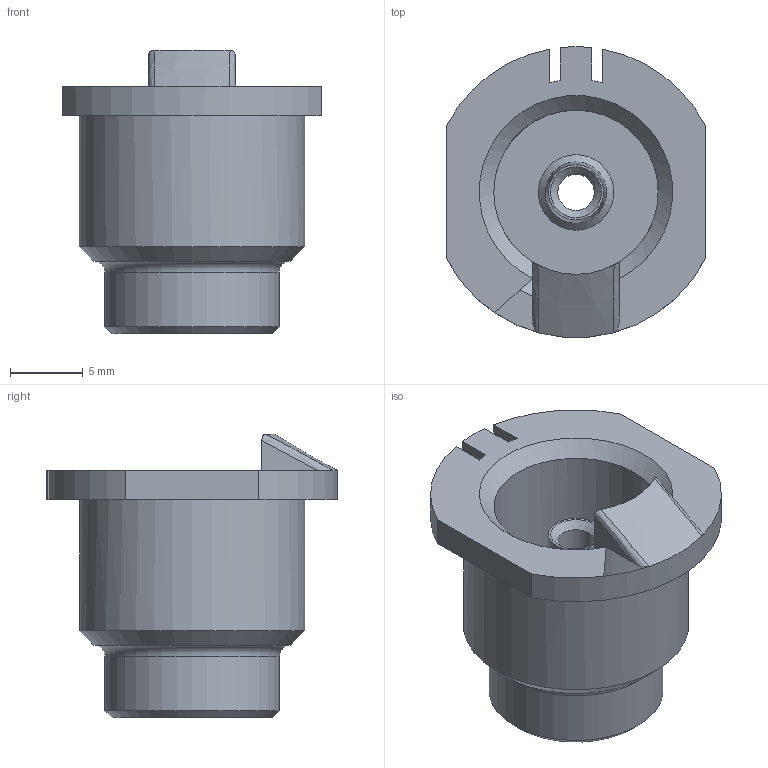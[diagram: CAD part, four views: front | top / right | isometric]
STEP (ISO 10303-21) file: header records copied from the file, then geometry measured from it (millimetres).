
FILE_DESCRIPTION(/* description */ (''),/* implementation_level */ '2;1');
FILE_NAME(/* name */ 'Fuse Base.step',/* time_stamp */ '2020-10-22T17:43:10-04:00',/* author */ (''),/* organization */ (''),/* preprocessor_version */ 'ST-DEVELOPER v18.1',/* originating_system */ 'Autodesk Translation Framework v9.3.0.1241',/* authorisation */ '');
FILE_SCHEMA (('AUTOMOTIVE_DESIGN { 1 0 10303 214 3 1 1 }'));
Length unit declared in the file: millimetre
Products named in the file (1): Fuse Base
Bounding box: 17.79 x 19.96 x 19.5 mm (x, y, z)
Volume: 1930.8 mm3; surface area: 1948.9 mm2
Topology: 1 solids, 1 shells, 44 faces, 111 edges, 72 vertices
Faces by surface type: plane 19, cylinder 12, cone 10, bspline 2, torus 1
Full cylindrical faces by diameter (mm): 2.5 x1, 3 x1, 4.191 x1, 6 x1, 11.3 x1, 12 x1, 15.5 x1
Entity records: 1494 total; most frequent: CARTESIAN_POINT 378, DIRECTION 235, ORIENTED_EDGE 222, EDGE_CURVE 111, AXIS2_PLACEMENT_3D 91, VERTEX_POINT 72, LINE 53, VECTOR 53
